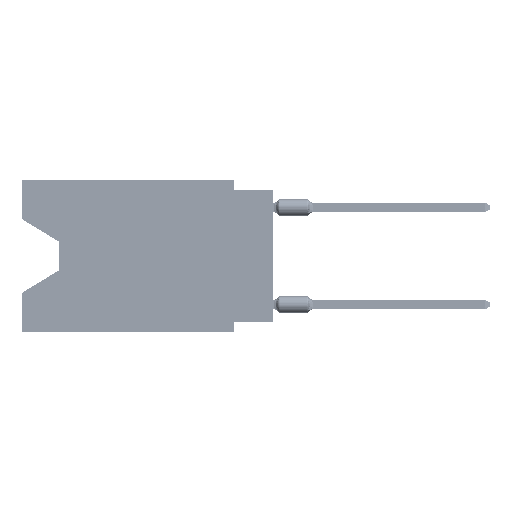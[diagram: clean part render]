
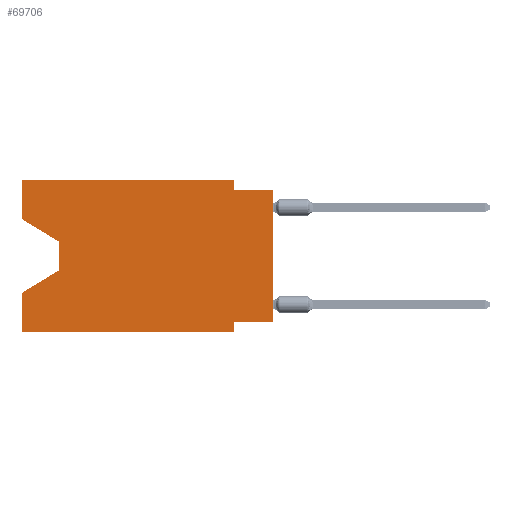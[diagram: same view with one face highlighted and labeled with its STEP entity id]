
A CAD part, left-side view. The second image highlights one B-rep face of the part: STEP entity #69706.
In plain terms, the highlighted planar face has unit normal (-1, 0, 0).
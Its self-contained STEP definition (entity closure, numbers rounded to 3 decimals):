
#55 = CARTESIAN_POINT ( 'NONE',  ( 0., 16.383, -7.36 ) ) ;
#895 = CARTESIAN_POINT ( 'NONE',  ( 0., 0., -0.635 ) ) ;
#987 = EDGE_CURVE ( 'NONE', #27449, #5443, #19932, .T. ) ;
#1367 = EDGE_CURVE ( 'NONE', #59820, #42417, #47123, .T. ) ;
#1627 = EDGE_CURVE ( 'NONE', #39934, #5443, #46317, .T. ) ;
#1932 = CARTESIAN_POINT ( 'NONE',  ( 0., 16.383, -2.546 ) ) ;
#2263 = ORIENTED_EDGE ( 'NONE', *, *, #1627, .F. ) ;
#4090 = VECTOR ( 'NONE', #59470, 1000. ) ;
#4679 = EDGE_CURVE ( 'NONE', #18834, #66220, #20392, .T. ) ;
#5176 = EDGE_CURVE ( 'NONE', #27449, #37642, #6714, .T. ) ;
#5272 = EDGE_LOOP ( 'NONE', ( #16430, #47301, #12438, #17172, #58808, #37786, #40848, #33510, #2263, #47993, #26661, #39886 ) ) ;
#5443 = VERTEX_POINT ( 'NONE', #60463 ) ;
#5673 = EDGE_CURVE ( 'NONE', #11178, #39934, #7354, .T. ) ;
#6714 = LINE ( 'NONE', #34329, #47595 ) ;
#7354 = LINE ( 'NONE', #14238, #30213 ) ;
#8611 = LINE ( 'NONE', #36237, #26789 ) ;
#9848 = DIRECTION ( 'NONE',  ( 0., 0., 1. ) ) ;
#10801 = LINE ( 'NONE', #49680, #53483 ) ;
#11078 = FACE_OUTER_BOUND ( 'NONE', #5272, .T. ) ;
#11178 = VERTEX_POINT ( 'NONE', #12098 ) ;
#11343 = CARTESIAN_POINT ( 'NONE',  ( 0., 2.54, -9.906 ) ) ;
#12088 = CARTESIAN_POINT ( 'NONE',  ( 0., 16.383, 0. ) ) ;
#12098 = CARTESIAN_POINT ( 'NONE',  ( 0., 2.54, 0. ) ) ;
#12438 = ORIENTED_EDGE ( 'NONE', *, *, #25875, .T. ) ;
#13893 = VECTOR ( 'NONE', #50341, 1000. ) ;
#14238 = CARTESIAN_POINT ( 'NONE',  ( 0., 2.54, 0. ) ) ;
#14547 = EDGE_CURVE ( 'NONE', #37642, #29111, #61148, .T. ) ;
#15116 = CARTESIAN_POINT ( 'NONE',  ( 0., 16.383, 0. ) ) ;
#16430 = ORIENTED_EDGE ( 'NONE', *, *, #65489, .T. ) ;
#17172 = ORIENTED_EDGE ( 'NONE', *, *, #1367, .F. ) ;
#17606 = DIRECTION ( 'NONE',  ( 0., -1., 0. ) ) ;
#18221 = CARTESIAN_POINT ( 'NONE',  ( 0., 13.97, -4.013 ) ) ;
#18277 = VERTEX_POINT ( 'NONE', #28542 ) ;
#18834 = VERTEX_POINT ( 'NONE', #1932 ) ;
#19932 = LINE ( 'NONE', #58463, #58613 ) ;
#20392 = LINE ( 'NONE', #37104, #63787 ) ;
#21207 = DIRECTION ( 'NONE',  ( 0., -1., 0. ) ) ;
#21658 = LINE ( 'NONE', #60910, #13893 ) ;
#25489 = DIRECTION ( 'NONE',  ( 0., 0., -1. ) ) ;
#25875 = EDGE_CURVE ( 'NONE', #18277, #42417, #21658, .T. ) ;
#26099 = DIRECTION ( 'NONE',  ( 0., 0., 1. ) ) ;
#26133 = VECTOR ( 'NONE', #21207, 1000. ) ;
#26300 = CARTESIAN_POINT ( 'NONE',  ( 0., 16.383, -9.906 ) ) ;
#26654 = LINE ( 'NONE', #26300, #26133 ) ;
#26661 = ORIENTED_EDGE ( 'NONE', *, *, #32315, .F. ) ;
#26789 = VECTOR ( 'NONE', #29710, 1000. ) ;
#27164 = CARTESIAN_POINT ( 'NONE',  ( 0., 2.54, -0.635 ) ) ;
#27449 = VERTEX_POINT ( 'NONE', #27729 ) ;
#27729 = CARTESIAN_POINT ( 'NONE',  ( 0., 0., -9.271 ) ) ;
#28426 = AXIS2_PLACEMENT_3D ( 'NONE', #44150, #33249, #55423 ) ;
#28542 = CARTESIAN_POINT ( 'NONE',  ( 0., 13.97, -5.893 ) ) ;
#29111 = VERTEX_POINT ( 'NONE', #64419 ) ;
#29710 = DIRECTION ( 'NONE',  ( 0., -0.855, -0.519 ) ) ;
#30213 = VECTOR ( 'NONE', #25489, 1000. ) ;
#32011 = VECTOR ( 'NONE', #17606, 1000. ) ;
#32315 = EDGE_CURVE ( 'NONE', #66220, #11178, #10801, .T. ) ;
#32891 = PLANE ( 'NONE',  #28426 ) ;
#33249 = DIRECTION ( 'NONE',  ( 1., 0., 0. ) ) ;
#33501 = DIRECTION ( 'NONE',  ( 0., 0., -1. ) ) ;
#33510 = ORIENTED_EDGE ( 'NONE', *, *, #987, .T. ) ;
#34329 = CARTESIAN_POINT ( 'NONE',  ( 0., 0., -9.271 ) ) ;
#36237 = CARTESIAN_POINT ( 'NONE',  ( 0., 16.383, -2.546 ) ) ;
#36636 = VERTEX_POINT ( 'NONE', #18221 ) ;
#37104 = CARTESIAN_POINT ( 'NONE',  ( 0., 16.383, 0. ) ) ;
#37642 = VERTEX_POINT ( 'NONE', #41994 ) ;
#37786 = ORIENTED_EDGE ( 'NONE', *, *, #14547, .F. ) ;
#39886 = ORIENTED_EDGE ( 'NONE', *, *, #4679, .F. ) ;
#39934 = VERTEX_POINT ( 'NONE', #27164 ) ;
#40848 = ORIENTED_EDGE ( 'NONE', *, *, #5176, .F. ) ;
#41994 = CARTESIAN_POINT ( 'NONE',  ( 0., 2.54, -9.271 ) ) ;
#42417 = VERTEX_POINT ( 'NONE', #55 ) ;
#43869 = DIRECTION ( 'NONE',  ( 0., -1., 0. ) ) ;
#43983 = CARTESIAN_POINT ( 'NONE',  ( 0., 16.383, -9.906 ) ) ;
#44150 = CARTESIAN_POINT ( 'NONE',  ( 0., 16.383, 0. ) ) ;
#46317 = LINE ( 'NONE', #895, #32011 ) ;
#47123 = LINE ( 'NONE', #15116, #4090 ) ;
#47301 = ORIENTED_EDGE ( 'NONE', *, *, #50769, .T. ) ;
#47595 = VECTOR ( 'NONE', #51423, 1000. ) ;
#47993 = ORIENTED_EDGE ( 'NONE', *, *, #5673, .F. ) ;
#49680 = CARTESIAN_POINT ( 'NONE',  ( 0., 16.383, 0. ) ) ;
#50341 = DIRECTION ( 'NONE',  ( 0., 0.855, -0.519 ) ) ;
#50769 = EDGE_CURVE ( 'NONE', #36636, #18277, #51329, .T. ) ;
#51329 = LINE ( 'NONE', #67332, #58007 ) ;
#51423 = DIRECTION ( 'NONE',  ( 0., 1., 0. ) ) ;
#53483 = VECTOR ( 'NONE', #43869, 1000. ) ;
#54738 = VECTOR ( 'NONE', #33501, 1000. ) ;
#55423 = DIRECTION ( 'NONE',  ( 0., 0., -1. ) ) ;
#56057 = DIRECTION ( 'NONE',  ( 0., 0., -1. ) ) ;
#57149 = EDGE_CURVE ( 'NONE', #59820, #29111, #26654, .T. ) ;
#58007 = VECTOR ( 'NONE', #56057, 1000. ) ;
#58463 = CARTESIAN_POINT ( 'NONE',  ( 0., 0., 0. ) ) ;
#58613 = VECTOR ( 'NONE', #26099, 1000. ) ;
#58808 = ORIENTED_EDGE ( 'NONE', *, *, #57149, .T. ) ;
#59470 = DIRECTION ( 'NONE',  ( 0., 0., 1. ) ) ;
#59820 = VERTEX_POINT ( 'NONE', #43983 ) ;
#60463 = CARTESIAN_POINT ( 'NONE',  ( 0., 0., -0.635 ) ) ;
#60910 = CARTESIAN_POINT ( 'NONE',  ( 0., 13.97, -5.893 ) ) ;
#61148 = LINE ( 'NONE', #11343, #54738 ) ;
#63787 = VECTOR ( 'NONE', #9848, 1000. ) ;
#64419 = CARTESIAN_POINT ( 'NONE',  ( 0., 2.54, -9.906 ) ) ;
#65489 = EDGE_CURVE ( 'NONE', #18834, #36636, #8611, .T. ) ;
#66220 = VERTEX_POINT ( 'NONE', #12088 ) ;
#67332 = CARTESIAN_POINT ( 'NONE',  ( 0., 13.97, -4.013 ) ) ;
#69706 = ADVANCED_FACE ( 'NONE', ( #11078 ), #32891, .F. ) ;
